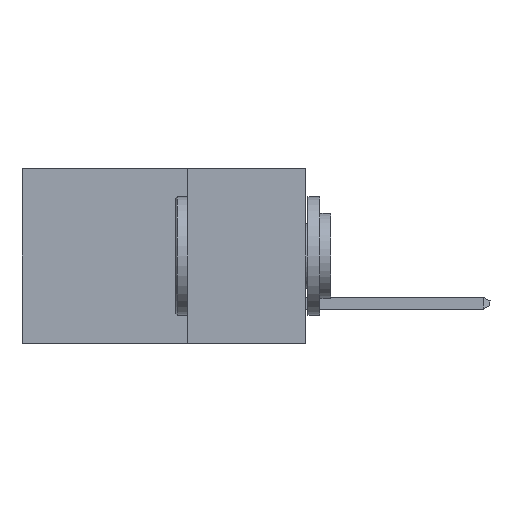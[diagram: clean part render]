
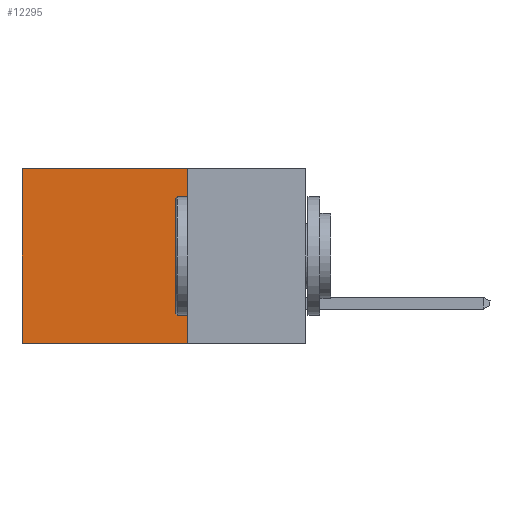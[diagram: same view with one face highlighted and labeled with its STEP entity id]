
A CAD part, left-side view. The second image highlights one B-rep face of the part: STEP entity #12295.
In plain terms, the highlighted planar face has unit normal (-1, 0, 0).
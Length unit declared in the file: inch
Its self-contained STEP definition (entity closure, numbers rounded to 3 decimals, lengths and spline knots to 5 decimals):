
#127 = EDGE_LOOP ( 'NONE', ( #9601, #17342, #4562, #11969 ) ) ;
#176 = AXIS2_PLACEMENT_3D ( 'NONE', #1984, #8039, #14008 ) ;
#880 = CARTESIAN_POINT ( 'NONE',  ( 0.298, 0.25, 0. ) ) ;
#1336 = EDGE_CURVE ( 'NONE', #4272, #18979, #14698, .T. ) ;
#1984 = CARTESIAN_POINT ( 'NONE',  ( 0.298, 0.25, 0. ) ) ;
#2688 = CARTESIAN_POINT ( 'NONE',  ( 0.298, 0.6, 0. ) ) ;
#3219 = EDGE_CURVE ( 'NONE', #9661, #18979, #8908, .T. ) ;
#4272 = VERTEX_POINT ( 'NONE', #5289 ) ;
#4562 = ORIENTED_EDGE ( 'NONE', *, *, #25739, .F. ) ;
#4901 = LINE ( 'NONE', #25289, #11121 ) ;
#5289 = CARTESIAN_POINT ( 'NONE',  ( 0.298, 0.25, -0.37 ) ) ;
#5379 = VECTOR ( 'NONE', #21405, 39.37008 ) ;
#6076 = VECTOR ( 'NONE', #20085, 39.37008 ) ;
#8039 = DIRECTION ( 'NONE',  ( 1., 0., 0. ) ) ;
#8084 = EDGE_CURVE ( 'NONE', #17944, #9661, #12673, .T. ) ;
#8908 = LINE ( 'NONE', #23963, #6076 ) ;
#8953 = CARTESIAN_POINT ( 'NONE',  ( 0.298, 0.25, 0. ) ) ;
#9327 = FACE_OUTER_BOUND ( 'NONE', #127, .T. ) ;
#9601 = ORIENTED_EDGE ( 'NONE', *, *, #3219, .T. ) ;
#9661 = VERTEX_POINT ( 'NONE', #2688 ) ;
#10352 = CARTESIAN_POINT ( 'NONE',  ( 0.298, 0.25, -0.37 ) ) ;
#11121 = VECTOR ( 'NONE', #13398, 39.37008 ) ;
#11969 = ORIENTED_EDGE ( 'NONE', *, *, #8084, .T. ) ;
#12295 = ADVANCED_FACE ( 'NONE', ( #9327 ), #13915, .F. ) ;
#12673 = LINE ( 'NONE', #880, #13279 ) ;
#13279 = VECTOR ( 'NONE', #14392, 39.37008 ) ;
#13398 = DIRECTION ( 'NONE',  ( 0., 0., -1. ) ) ;
#13915 = PLANE ( 'NONE',  #176 ) ;
#14008 = DIRECTION ( 'NONE',  ( 0., 0., -1. ) ) ;
#14392 = DIRECTION ( 'NONE',  ( 0., 1., 0. ) ) ;
#14698 = LINE ( 'NONE', #10352, #5379 ) ;
#17342 = ORIENTED_EDGE ( 'NONE', *, *, #1336, .F. ) ;
#17944 = VERTEX_POINT ( 'NONE', #8953 ) ;
#18979 = VERTEX_POINT ( 'NONE', #20599 ) ;
#20085 = DIRECTION ( 'NONE',  ( 0., 0., -1. ) ) ;
#20599 = CARTESIAN_POINT ( 'NONE',  ( 0.298, 0.6, -0.37 ) ) ;
#21405 = DIRECTION ( 'NONE',  ( 0., 1., 0. ) ) ;
#23963 = CARTESIAN_POINT ( 'NONE',  ( 0.298, 0.6, 0. ) ) ;
#25289 = CARTESIAN_POINT ( 'NONE',  ( 0.298, 0.25, 0. ) ) ;
#25739 = EDGE_CURVE ( 'NONE', #17944, #4272, #4901, .T. ) ;
